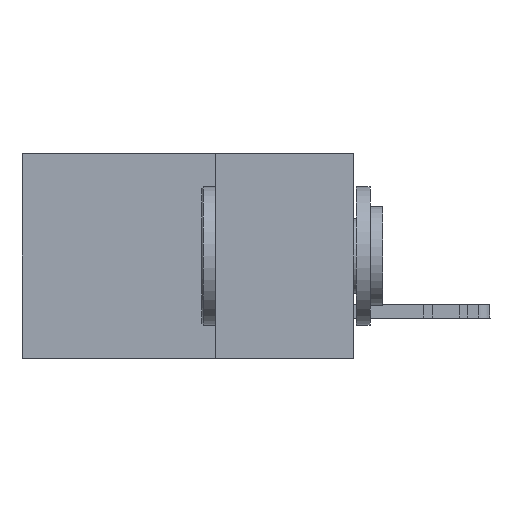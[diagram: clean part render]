
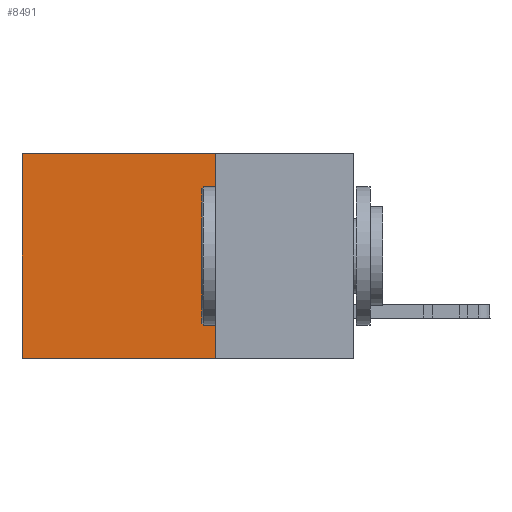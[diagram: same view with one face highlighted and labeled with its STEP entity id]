
A CAD part, left-side view. The second image highlights one B-rep face of the part: STEP entity #8491.
In plain terms, the highlighted planar face has unit normal (-1, 0, 0).
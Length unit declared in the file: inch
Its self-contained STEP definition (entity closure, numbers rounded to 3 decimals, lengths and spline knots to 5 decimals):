
#957 = VECTOR ( 'NONE', #22793, 39.37008 ) ;
#2932 = DIRECTION ( 'NONE',  ( 0., 0., -1. ) ) ;
#3522 = VERTEX_POINT ( 'NONE', #15032 ) ;
#5418 = DIRECTION ( 'NONE',  ( 0., 0., -1. ) ) ;
#5497 = AXIS2_PLACEMENT_3D ( 'NONE', #28037, #24469, #31279 ) ;
#5964 = VERTEX_POINT ( 'NONE', #28241 ) ;
#6119 = ORIENTED_EDGE ( 'NONE', *, *, #41760, .T. ) ;
#7522 = LINE ( 'NONE', #29885, #39459 ) ;
#8485 = ORIENTED_EDGE ( 'NONE', *, *, #13210, .F. ) ;
#8491 = ADVANCED_FACE ( 'NONE', ( #30284 ), #20752, .F. ) ;
#9945 = EDGE_LOOP ( 'NONE', ( #34198, #16987, #8485, #6119 ) ) ;
#13210 = EDGE_CURVE ( 'NONE', #14457, #5964, #40171, .T. ) ;
#14457 = VERTEX_POINT ( 'NONE', #39855 ) ;
#14533 = VECTOR ( 'NONE', #25927, 39.37008 ) ;
#15032 = CARTESIAN_POINT ( 'NONE',  ( 0.2875, 0.6, -0.37 ) ) ;
#16313 = LINE ( 'NONE', #32421, #957 ) ;
#16987 = ORIENTED_EDGE ( 'NONE', *, *, #17713, .F. ) ;
#17713 = EDGE_CURVE ( 'NONE', #5964, #3522, #36338, .T. ) ;
#17864 = CARTESIAN_POINT ( 'NONE',  ( 0.2875, 0.25, 0. ) ) ;
#18222 = EDGE_CURVE ( 'NONE', #42188, #3522, #7522, .T. ) ;
#20241 = CARTESIAN_POINT ( 'NONE',  ( 0.2875, 0.25, -0.37 ) ) ;
#20752 = PLANE ( 'NONE',  #5497 ) ;
#22617 = VECTOR ( 'NONE', #5418, 39.37008 ) ;
#22793 = DIRECTION ( 'NONE',  ( 0., 1., 0. ) ) ;
#24469 = DIRECTION ( 'NONE',  ( 1., 0., 0. ) ) ;
#25927 = DIRECTION ( 'NONE',  ( 0., 1., 0. ) ) ;
#26927 = CARTESIAN_POINT ( 'NONE',  ( 0.2875, 0.6, 0. ) ) ;
#28037 = CARTESIAN_POINT ( 'NONE',  ( 0.2875, 0.25, 0. ) ) ;
#28241 = CARTESIAN_POINT ( 'NONE',  ( 0.2875, 0.25, -0.37 ) ) ;
#29885 = CARTESIAN_POINT ( 'NONE',  ( 0.2875, 0.6, 0. ) ) ;
#30284 = FACE_OUTER_BOUND ( 'NONE', #9945, .T. ) ;
#31279 = DIRECTION ( 'NONE',  ( 0., 0., -1. ) ) ;
#32421 = CARTESIAN_POINT ( 'NONE',  ( 0.2875, 0.25, 0. ) ) ;
#34198 = ORIENTED_EDGE ( 'NONE', *, *, #18222, .T. ) ;
#36338 = LINE ( 'NONE', #20241, #14533 ) ;
#39459 = VECTOR ( 'NONE', #2932, 39.37008 ) ;
#39855 = CARTESIAN_POINT ( 'NONE',  ( 0.2875, 0.25, 0. ) ) ;
#40171 = LINE ( 'NONE', #17864, #22617 ) ;
#41760 = EDGE_CURVE ( 'NONE', #14457, #42188, #16313, .T. ) ;
#42188 = VERTEX_POINT ( 'NONE', #26927 ) ;
